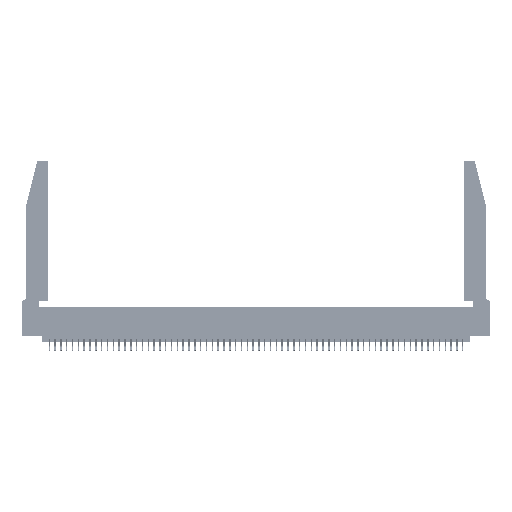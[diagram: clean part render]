
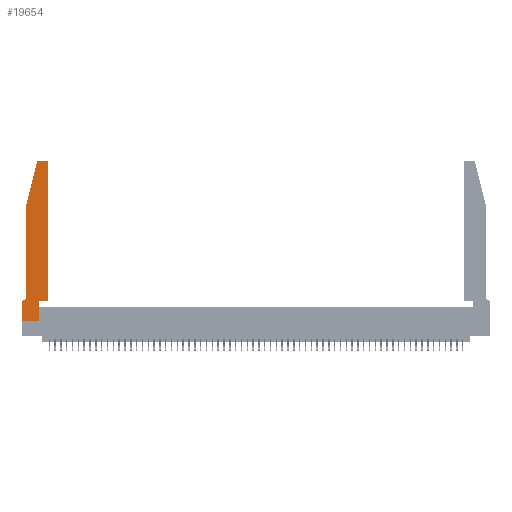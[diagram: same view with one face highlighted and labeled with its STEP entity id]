
A CAD part, top view. The second image highlights one B-rep face of the part: STEP entity #19654.
In plain terms, the highlighted planar face has unit normal (0, 0, 1).
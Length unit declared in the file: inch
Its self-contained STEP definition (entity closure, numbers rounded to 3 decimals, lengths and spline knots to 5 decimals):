
#1690 = EDGE_LOOP ( 'NONE', ( #13071, #15301, #17854, #33601, #24892, #33040, #10823, #57392, #39896, #51180, #27124, #45857 ) ) ;
#2077 = LINE ( 'NONE', #20015, #36263 ) ;
#2166 = DIRECTION ( 'NONE',  ( 0., 1., 0. ) ) ;
#2175 = LINE ( 'NONE', #22283, #36349 ) ;
#2569 = VERTEX_POINT ( 'NONE', #10662 ) ;
#5280 = AXIS2_PLACEMENT_3D ( 'NONE', #43316, #56836, #30446 ) ;
#5863 = DIRECTION ( 'NONE',  ( 0., 0., 1. ) ) ;
#7449 = CIRCLE ( 'NONE', #38753, 0.03 ) ;
#7576 = EDGE_CURVE ( 'NONE', #2569, #14860, #33755, .T. ) ;
#8895 = VECTOR ( 'NONE', #23290, 39.37008 ) ;
#9907 = CIRCLE ( 'NONE', #30937, 0.03 ) ;
#10141 = VECTOR ( 'NONE', #50325, 39.37008 ) ;
#10503 = DIRECTION ( 'NONE',  ( 0., 0., -1. ) ) ;
#10662 = CARTESIAN_POINT ( 'NONE',  ( 0.25487, 2.72718, 0.37 ) ) ;
#10823 = ORIENTED_EDGE ( 'NONE', *, *, #17861, .T. ) ;
#10833 = CARTESIAN_POINT ( 'NONE',  ( 0.0055, 0.35, 0.37 ) ) ;
#11588 = DIRECTION ( 'NONE',  ( 1., 0., 0. ) ) ;
#11645 = CARTESIAN_POINT ( 'NONE',  ( 0., 0.35, 0.37 ) ) ;
#11961 = DIRECTION ( 'NONE',  ( 0., 1., 0. ) ) ;
#13071 = ORIENTED_EDGE ( 'NONE', *, *, #41404, .T. ) ;
#13359 = EDGE_CURVE ( 'NONE', #38683, #22949, #33688, .T. ) ;
#13448 = EDGE_CURVE ( 'NONE', #22949, #31545, #19162, .T. ) ;
#14727 = EDGE_CURVE ( 'NONE', #51406, #2569, #9907, .T. ) ;
#14860 = VERTEX_POINT ( 'NONE', #20621 ) ;
#15301 = ORIENTED_EDGE ( 'NONE', *, *, #14727, .T. ) ;
#16051 = CARTESIAN_POINT ( 'NONE',  ( 0., 0., 0.37 ) ) ;
#16917 = VERTEX_POINT ( 'NONE', #30266 ) ;
#17854 = ORIENTED_EDGE ( 'NONE', *, *, #7576, .T. ) ;
#17861 = EDGE_CURVE ( 'NONE', #31545, #31327, #44217, .T. ) ;
#17922 = EDGE_CURVE ( 'NONE', #25414, #18508, #7449, .T. ) ;
#18508 = VERTEX_POINT ( 'NONE', #49051 ) ;
#18831 = CARTESIAN_POINT ( 'NONE',  ( 0., 0., 0.37 ) ) ;
#19092 = CARTESIAN_POINT ( 'NONE',  ( 0.284, 2.72, 0.37 ) ) ;
#19162 = LINE ( 'NONE', #28755, #51597 ) ;
#19248 = CARTESIAN_POINT ( 'NONE',  ( 0., 0., 0.37 ) ) ;
#19654 = ADVANCED_FACE ( 'NONE', ( #22800 ), #26002, .T. ) ;
#20015 = CARTESIAN_POINT ( 'NONE',  ( 0.0755, 2., 0.37 ) ) ;
#20194 = CARTESIAN_POINT ( 'NONE',  ( 0.4505, 2.72, 0.37 ) ) ;
#20621 = CARTESIAN_POINT ( 'NONE',  ( 0.0755, 2., 0.37 ) ) ;
#21776 = EDGE_CURVE ( 'NONE', #28737, #16917, #34943, .T. ) ;
#22283 = CARTESIAN_POINT ( 'NONE',  ( 0.2605, 2.75, 0.37 ) ) ;
#22800 = FACE_OUTER_BOUND ( 'NONE', #1690, .T. ) ;
#22949 = VERTEX_POINT ( 'NONE', #10833 ) ;
#23290 = DIRECTION ( 'NONE',  ( 0., -1., 0. ) ) ;
#23529 = DIRECTION ( 'NONE',  ( 1., 0., 0. ) ) ;
#24831 = VECTOR ( 'NONE', #2166, 39.37008 ) ;
#24892 = ORIENTED_EDGE ( 'NONE', *, *, #13359, .T. ) ;
#24949 = DIRECTION ( 'NONE',  ( 1., 0., 0. ) ) ;
#25414 = VERTEX_POINT ( 'NONE', #20194 ) ;
#25647 = CARTESIAN_POINT ( 'NONE',  ( 0.284, 2.75, 0.37 ) ) ;
#26002 = PLANE ( 'NONE',  #5280 ) ;
#26241 = VECTOR ( 'NONE', #11961, 39.37008 ) ;
#27124 = ORIENTED_EDGE ( 'NONE', *, *, #49208, .T. ) ;
#28737 = VERTEX_POINT ( 'NONE', #50119 ) ;
#28738 = LINE ( 'NONE', #16051, #53549 ) ;
#28755 = CARTESIAN_POINT ( 'NONE',  ( 0.0755, 0.35, 0.37 ) ) ;
#28866 = EDGE_CURVE ( 'NONE', #14860, #38683, #2077, .T. ) ;
#30266 = CARTESIAN_POINT ( 'NONE',  ( 0.4505, 0.35, 0.37 ) ) ;
#30446 = DIRECTION ( 'NONE',  ( 1., 0., 0. ) ) ;
#30937 = AXIS2_PLACEMENT_3D ( 'NONE', #19092, #49941, #23529 ) ;
#31327 = VERTEX_POINT ( 'NONE', #19248 ) ;
#31545 = VERTEX_POINT ( 'NONE', #11645 ) ;
#32175 = VECTOR ( 'NONE', #11588, 39.37008 ) ;
#32542 = CARTESIAN_POINT ( 'NONE',  ( 0.4205, 2.72, 0.37 ) ) ;
#32787 = CARTESIAN_POINT ( 'NONE',  ( 0.0755, 2., 0.37 ) ) ;
#33040 = ORIENTED_EDGE ( 'NONE', *, *, #13448, .T. ) ;
#33601 = ORIENTED_EDGE ( 'NONE', *, *, #28866, .T. ) ;
#33688 = CIRCLE ( 'NONE', #47116, 0.07 ) ;
#33755 = LINE ( 'NONE', #32787, #10141 ) ;
#34943 = LINE ( 'NONE', #42460, #32175 ) ;
#36263 = VECTOR ( 'NONE', #46422, 39.37008 ) ;
#36349 = VECTOR ( 'NONE', #39997, 39.37008 ) ;
#36965 = DIRECTION ( 'NONE',  ( 1., 0., 0. ) ) ;
#37047 = CARTESIAN_POINT ( 'NONE',  ( 0.0055, 0.42, 0.37 ) ) ;
#37992 = LINE ( 'NONE', #55971, #26241 ) ;
#38683 = VERTEX_POINT ( 'NONE', #53644 ) ;
#38753 = AXIS2_PLACEMENT_3D ( 'NONE', #32542, #5863, #36965 ) ;
#39896 = ORIENTED_EDGE ( 'NONE', *, *, #48783, .T. ) ;
#39997 = DIRECTION ( 'NONE',  ( -1., 0., 0. ) ) ;
#41404 = EDGE_CURVE ( 'NONE', #18508, #51406, #2175, .T. ) ;
#41432 = DIRECTION ( 'NONE',  ( -1., 0., 0. ) ) ;
#41809 = EDGE_CURVE ( 'NONE', #31327, #45555, #28738, .T. ) ;
#42460 = CARTESIAN_POINT ( 'NONE',  ( 0.4505, 0.35, 0.37 ) ) ;
#43316 = CARTESIAN_POINT ( 'NONE',  ( 0., 0.35, 0.37 ) ) ;
#44217 = LINE ( 'NONE', #18831, #8895 ) ;
#45555 = VERTEX_POINT ( 'NONE', #47267 ) ;
#45857 = ORIENTED_EDGE ( 'NONE', *, *, #17922, .T. ) ;
#46422 = DIRECTION ( 'NONE',  ( 0., -1., 0. ) ) ;
#47116 = AXIS2_PLACEMENT_3D ( 'NONE', #37047, #10503, #41432 ) ;
#47267 = CARTESIAN_POINT ( 'NONE',  ( 0.2865, 0., 0.37 ) ) ;
#48262 = LINE ( 'NONE', #55355, #24831 ) ;
#48783 = EDGE_CURVE ( 'NONE', #45555, #28737, #37992, .T. ) ;
#49051 = CARTESIAN_POINT ( 'NONE',  ( 0.4205, 2.75, 0.37 ) ) ;
#49208 = EDGE_CURVE ( 'NONE', #16917, #25414, #48262, .T. ) ;
#49941 = DIRECTION ( 'NONE',  ( 0., 0., 1. ) ) ;
#50119 = CARTESIAN_POINT ( 'NONE',  ( 0.2865, 0.35, 0.37 ) ) ;
#50325 = DIRECTION ( 'NONE',  ( -0.239, -0.971, 0. ) ) ;
#50732 = DIRECTION ( 'NONE',  ( -1., 0., 0. ) ) ;
#51180 = ORIENTED_EDGE ( 'NONE', *, *, #21776, .T. ) ;
#51406 = VERTEX_POINT ( 'NONE', #25647 ) ;
#51597 = VECTOR ( 'NONE', #50732, 39.37008 ) ;
#53549 = VECTOR ( 'NONE', #24949, 39.37008 ) ;
#53644 = CARTESIAN_POINT ( 'NONE',  ( 0.0755, 0.42, 0.37 ) ) ;
#55355 = CARTESIAN_POINT ( 'NONE',  ( 0.4505, 0.35, 0.37 ) ) ;
#55971 = CARTESIAN_POINT ( 'NONE',  ( 0.2865, 0.35, 0.37 ) ) ;
#56836 = DIRECTION ( 'NONE',  ( 0., 0., 1. ) ) ;
#57392 = ORIENTED_EDGE ( 'NONE', *, *, #41809, .T. ) ;
